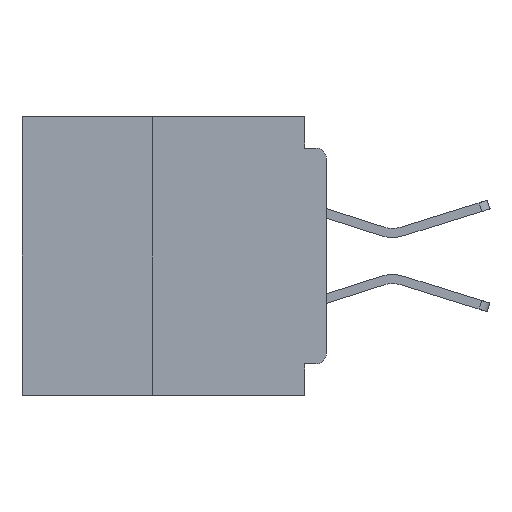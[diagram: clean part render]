
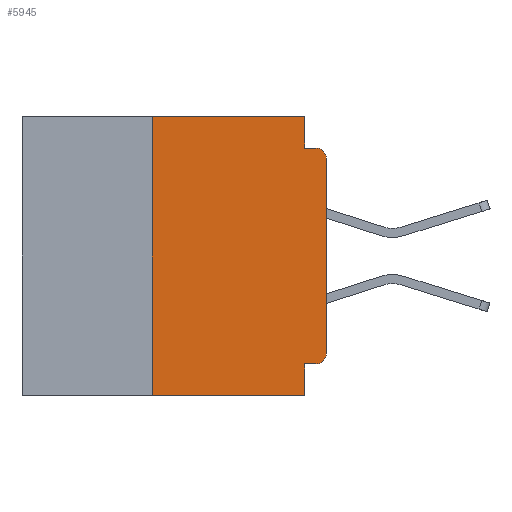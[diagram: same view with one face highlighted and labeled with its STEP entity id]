
A CAD part, left-side view. The second image highlights one B-rep face of the part: STEP entity #5945.
In plain terms, the highlighted planar face has unit normal (-1, 0, 0).
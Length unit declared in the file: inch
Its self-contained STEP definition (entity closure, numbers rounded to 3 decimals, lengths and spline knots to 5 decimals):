
#727 = EDGE_CURVE ( 'NONE', #26084, #33945, #36779, .T. ) ;
#859 = EDGE_CURVE ( 'NONE', #11402, #48827, #51174, .T. ) ;
#3413 = ORIENTED_EDGE ( 'NONE', *, *, #32048, .F. ) ;
#3482 = VERTEX_POINT ( 'NONE', #47642 ) ;
#3700 = CARTESIAN_POINT ( 'NONE',  ( 0., 0.25, -0.4 ) ) ;
#5395 = CARTESIAN_POINT ( 'NONE',  ( 0., 0.437, -0.4 ) ) ;
#5945 = ADVANCED_FACE ( 'NONE', ( #7432 ), #29139, .F. ) ;
#6941 = CARTESIAN_POINT ( 'NONE',  ( 0., 0.015, -0.045 ) ) ;
#7432 = FACE_OUTER_BOUND ( 'NONE', #18548, .T. ) ;
#8479 = DIRECTION ( 'NONE',  ( 0., -1., 0. ) ) ;
#9266 = VECTOR ( 'NONE', #8479, 39.37008 ) ;
#9295 = DIRECTION ( 'NONE',  ( 0., 0., 1. ) ) ;
#9467 = VERTEX_POINT ( 'NONE', #24817 ) ;
#10827 = CARTESIAN_POINT ( 'NONE',  ( 0., 0.031, -0.4 ) ) ;
#11348 = EDGE_CURVE ( 'NONE', #9467, #14325, #50033, .T. ) ;
#11402 = VERTEX_POINT ( 'NONE', #48487 ) ;
#11466 = VECTOR ( 'NONE', #9295, 39.37008 ) ;
#11698 = EDGE_CURVE ( 'NONE', #40441, #41318, #53908, .T. ) ;
#12365 = ORIENTED_EDGE ( 'NONE', *, *, #859, .T. ) ;
#12388 = DIRECTION ( 'NONE',  ( 0., 0., -1. ) ) ;
#12448 = VECTOR ( 'NONE', #24803, 39.37008 ) ;
#13316 = ORIENTED_EDGE ( 'NONE', *, *, #39587, .T. ) ;
#14325 = VERTEX_POINT ( 'NONE', #6941 ) ;
#14438 = VECTOR ( 'NONE', #53027, 39.37008 ) ;
#15915 = EDGE_CURVE ( 'NONE', #3482, #14325, #17972, .T. ) ;
#16581 = VECTOR ( 'NONE', #48124, 39.37008 ) ;
#16802 = VECTOR ( 'NONE', #36867, 39.37008 ) ;
#17972 = CIRCLE ( 'NONE', #36621, 0.015 ) ;
#18548 = EDGE_LOOP ( 'NONE', ( #13316, #27166, #19591, #3413, #22138, #30662, #42571, #50587, #34933, #12365 ) ) ;
#19591 = ORIENTED_EDGE ( 'NONE', *, *, #11348, .F. ) ;
#19843 = CARTESIAN_POINT ( 'NONE',  ( 0., 0.031, -0.355 ) ) ;
#20576 = DIRECTION ( 'NONE',  ( -1., 0., 0. ) ) ;
#20967 = CARTESIAN_POINT ( 'NONE',  ( 0., 0.437, 0. ) ) ;
#21324 = LINE ( 'NONE', #38679, #11466 ) ;
#21484 = DIRECTION ( 'NONE',  ( -1., 0., 0. ) ) ;
#22138 = ORIENTED_EDGE ( 'NONE', *, *, #11698, .F. ) ;
#22341 = LINE ( 'NONE', #35434, #30920 ) ;
#23602 = LINE ( 'NONE', #3700, #12448 ) ;
#24097 = CARTESIAN_POINT ( 'NONE',  ( 0., 0.031, 0. ) ) ;
#24803 = DIRECTION ( 'NONE',  ( 0., 0., 1. ) ) ;
#24817 = CARTESIAN_POINT ( 'NONE',  ( 0., 0.031, -0.045 ) ) ;
#24881 = CARTESIAN_POINT ( 'NONE',  ( 0., 0.437, 0. ) ) ;
#24984 = EDGE_CURVE ( 'NONE', #33196, #40441, #23602, .T. ) ;
#26065 = LINE ( 'NONE', #49324, #16802 ) ;
#26084 = VERTEX_POINT ( 'NONE', #19843 ) ;
#27166 = ORIENTED_EDGE ( 'NONE', *, *, #15915, .T. ) ;
#28196 = AXIS2_PLACEMENT_3D ( 'NONE', #24881, #37562, #12388 ) ;
#28572 = EDGE_CURVE ( 'NONE', #11402, #26084, #26065, .T. ) ;
#29139 = PLANE ( 'NONE',  #28196 ) ;
#30104 = VECTOR ( 'NONE', #30595, 39.37008 ) ;
#30595 = DIRECTION ( 'NONE',  ( 0., -1., 0. ) ) ;
#30662 = ORIENTED_EDGE ( 'NONE', *, *, #24984, .F. ) ;
#30920 = VECTOR ( 'NONE', #51906, 39.37008 ) ;
#31393 = LINE ( 'NONE', #5395, #30104 ) ;
#32048 = EDGE_CURVE ( 'NONE', #41318, #9467, #22341, .T. ) ;
#33196 = VERTEX_POINT ( 'NONE', #47045 ) ;
#33945 = VERTEX_POINT ( 'NONE', #10827 ) ;
#34933 = ORIENTED_EDGE ( 'NONE', *, *, #28572, .F. ) ;
#35406 = CARTESIAN_POINT ( 'NONE',  ( 0., 0., -0.34 ) ) ;
#35434 = CARTESIAN_POINT ( 'NONE',  ( 0., 0.031, 0. ) ) ;
#36621 = AXIS2_PLACEMENT_3D ( 'NONE', #46624, #21484, #50832 ) ;
#36779 = LINE ( 'NONE', #48813, #14438 ) ;
#36867 = DIRECTION ( 'NONE',  ( 0., 1., 0. ) ) ;
#37562 = DIRECTION ( 'NONE',  ( 1., 0., 0. ) ) ;
#38679 = CARTESIAN_POINT ( 'NONE',  ( 0., 0., 0. ) ) ;
#39587 = EDGE_CURVE ( 'NONE', #48827, #3482, #21324, .T. ) ;
#40441 = VERTEX_POINT ( 'NONE', #43114 ) ;
#41318 = VERTEX_POINT ( 'NONE', #24097 ) ;
#42571 = ORIENTED_EDGE ( 'NONE', *, *, #42925, .T. ) ;
#42925 = EDGE_CURVE ( 'NONE', #33196, #33945, #31393, .T. ) ;
#43114 = CARTESIAN_POINT ( 'NONE',  ( 0., 0.25, 0. ) ) ;
#43936 = CARTESIAN_POINT ( 'NONE',  ( 0., 0., -0.045 ) ) ;
#45696 = CARTESIAN_POINT ( 'NONE',  ( 0., 0.015, -0.34 ) ) ;
#46624 = CARTESIAN_POINT ( 'NONE',  ( 0., 0.015, -0.06 ) ) ;
#47045 = CARTESIAN_POINT ( 'NONE',  ( 0., 0.25, -0.4 ) ) ;
#47642 = CARTESIAN_POINT ( 'NONE',  ( 0., 0., -0.06 ) ) ;
#48124 = DIRECTION ( 'NONE',  ( 0., -1., 0. ) ) ;
#48487 = CARTESIAN_POINT ( 'NONE',  ( 0., 0.015, -0.355 ) ) ;
#48813 = CARTESIAN_POINT ( 'NONE',  ( 0., 0.031, -0.4 ) ) ;
#48827 = VERTEX_POINT ( 'NONE', #35406 ) ;
#49324 = CARTESIAN_POINT ( 'NONE',  ( 0., 0., -0.355 ) ) ;
#49771 = AXIS2_PLACEMENT_3D ( 'NONE', #45696, #20576, #49913 ) ;
#49913 = DIRECTION ( 'NONE',  ( 0., 0., -1. ) ) ;
#50033 = LINE ( 'NONE', #43936, #16581 ) ;
#50587 = ORIENTED_EDGE ( 'NONE', *, *, #727, .F. ) ;
#50832 = DIRECTION ( 'NONE',  ( 0., 0., -1. ) ) ;
#51174 = CIRCLE ( 'NONE', #49771, 0.015 ) ;
#51906 = DIRECTION ( 'NONE',  ( 0., 0., -1. ) ) ;
#53027 = DIRECTION ( 'NONE',  ( 0., 0., -1. ) ) ;
#53908 = LINE ( 'NONE', #20967, #9266 ) ;
